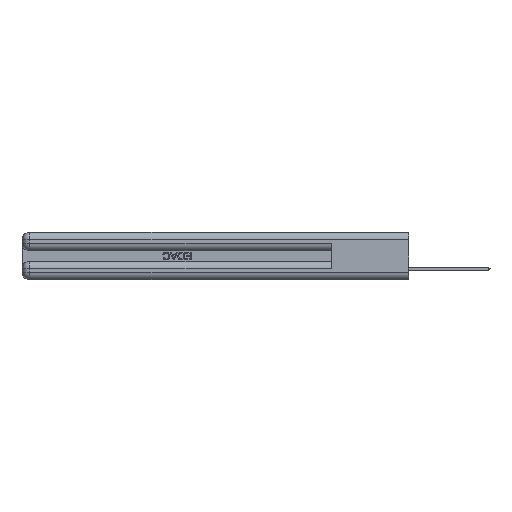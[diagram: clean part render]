
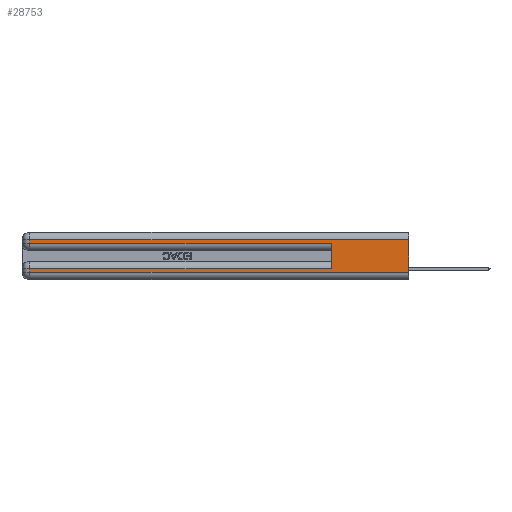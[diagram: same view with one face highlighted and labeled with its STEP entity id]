
A CAD part, left-side view. The second image highlights one B-rep face of the part: STEP entity #28753.
In plain terms, the highlighted planar face has unit normal (-1, 0, 0).
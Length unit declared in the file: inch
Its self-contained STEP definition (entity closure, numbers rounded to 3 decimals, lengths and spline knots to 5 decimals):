
#1187 = CARTESIAN_POINT ( 'NONE',  ( 0., 2.94, 0.31 ) ) ;
#1311 = VECTOR ( 'NONE', #47342, 39.37008 ) ;
#2061 = VERTEX_POINT ( 'NONE', #22111 ) ;
#3007 = CARTESIAN_POINT ( 'NONE',  ( 0., 0., 0.31 ) ) ;
#4517 = LINE ( 'NONE', #20306, #35977 ) ;
#5381 = ORIENTED_EDGE ( 'NONE', *, *, #28192, .T. ) ;
#7694 = DIRECTION ( 'NONE',  ( 0., 1., 0. ) ) ;
#9049 = EDGE_CURVE ( 'NONE', #15280, #13656, #18697, .T. ) ;
#9583 = EDGE_CURVE ( 'NONE', #20522, #40285, #17499, .T. ) ;
#11757 = PLANE ( 'NONE',  #12624 ) ;
#12578 = VECTOR ( 'NONE', #39625, 39.37008 ) ;
#12600 = EDGE_LOOP ( 'NONE', ( #22124, #5381, #37845, #44652, #40522, #27484, #21567, #27332 ) ) ;
#12624 = AXIS2_PLACEMENT_3D ( 'NONE', #39375, #23442, #51033 ) ;
#12992 = VERTEX_POINT ( 'NONE', #1187 ) ;
#13656 = VERTEX_POINT ( 'NONE', #49601 ) ;
#13977 = LINE ( 'NONE', #23666, #30680 ) ;
#15280 = VERTEX_POINT ( 'NONE', #34866 ) ;
#15989 = DIRECTION ( 'NONE',  ( 0., -1., 0. ) ) ;
#17499 = LINE ( 'NONE', #47185, #12578 ) ;
#18697 = LINE ( 'NONE', #21421, #29178 ) ;
#19286 = CARTESIAN_POINT ( 'NONE',  ( 0., 0., 0.06 ) ) ;
#20298 = CARTESIAN_POINT ( 'NONE',  ( 0., 0., 0.06 ) ) ;
#20306 = CARTESIAN_POINT ( 'NONE',  ( 0., 2.94, 0.37 ) ) ;
#20480 = DIRECTION ( 'NONE',  ( 0., 0., -1. ) ) ;
#20522 = VERTEX_POINT ( 'NONE', #38271 ) ;
#21421 = CARTESIAN_POINT ( 'NONE',  ( 0., 0., 0.085 ) ) ;
#21567 = ORIENTED_EDGE ( 'NONE', *, *, #30758, .T. ) ;
#22111 = CARTESIAN_POINT ( 'NONE',  ( 0., 2.94, 0.06 ) ) ;
#22124 = ORIENTED_EDGE ( 'NONE', *, *, #33357, .F. ) ;
#22220 = LINE ( 'NONE', #31991, #1311 ) ;
#22892 = EDGE_CURVE ( 'NONE', #15280, #40285, #22220, .T. ) ;
#23376 = VERTEX_POINT ( 'NONE', #3007 ) ;
#23442 = DIRECTION ( 'NONE',  ( 1., 0., 0. ) ) ;
#23666 = CARTESIAN_POINT ( 'NONE',  ( 0., 0., 0.31 ) ) ;
#24849 = DIRECTION ( 'NONE',  ( 0., 0., -1. ) ) ;
#25386 = DIRECTION ( 'NONE',  ( 0., 1., 0. ) ) ;
#25401 = CARTESIAN_POINT ( 'NONE',  ( 0., 2.94, 0.37 ) ) ;
#27332 = ORIENTED_EDGE ( 'NONE', *, *, #34290, .T. ) ;
#27484 = ORIENTED_EDGE ( 'NONE', *, *, #9049, .T. ) ;
#27805 = CARTESIAN_POINT ( 'NONE',  ( 0., 0.6, 0.285 ) ) ;
#28192 = EDGE_CURVE ( 'NONE', #23376, #12992, #13977, .T. ) ;
#28753 = ADVANCED_FACE ( 'NONE', ( #34325 ), #11757, .F. ) ;
#29178 = VECTOR ( 'NONE', #25386, 39.37008 ) ;
#29346 = CARTESIAN_POINT ( 'NONE',  ( 0., 0., 0.37 ) ) ;
#29542 = EDGE_CURVE ( 'NONE', #12992, #20522, #33020, .T. ) ;
#30680 = VECTOR ( 'NONE', #7694, 39.37008 ) ;
#30758 = EDGE_CURVE ( 'NONE', #13656, #2061, #4517, .T. ) ;
#31773 = VECTOR ( 'NONE', #45128, 39.37008 ) ;
#31991 = CARTESIAN_POINT ( 'NONE',  ( 0., 0.6, 0.145 ) ) ;
#33020 = LINE ( 'NONE', #25401, #31773 ) ;
#33357 = EDGE_CURVE ( 'NONE', #23376, #49647, #34187, .T. ) ;
#34187 = LINE ( 'NONE', #29346, #46556 ) ;
#34290 = EDGE_CURVE ( 'NONE', #2061, #49647, #49668, .T. ) ;
#34325 = FACE_OUTER_BOUND ( 'NONE', #12600, .T. ) ;
#34866 = CARTESIAN_POINT ( 'NONE',  ( 0., 0.6, 0.085 ) ) ;
#35977 = VECTOR ( 'NONE', #20480, 39.37008 ) ;
#37845 = ORIENTED_EDGE ( 'NONE', *, *, #29542, .T. ) ;
#38271 = CARTESIAN_POINT ( 'NONE',  ( 0., 2.94, 0.285 ) ) ;
#39375 = CARTESIAN_POINT ( 'NONE',  ( 0., 0., 0.37 ) ) ;
#39625 = DIRECTION ( 'NONE',  ( 0., -1., 0. ) ) ;
#39869 = VECTOR ( 'NONE', #15989, 39.37008 ) ;
#40285 = VERTEX_POINT ( 'NONE', #27805 ) ;
#40522 = ORIENTED_EDGE ( 'NONE', *, *, #22892, .F. ) ;
#44652 = ORIENTED_EDGE ( 'NONE', *, *, #9583, .T. ) ;
#45128 = DIRECTION ( 'NONE',  ( 0., 0., -1. ) ) ;
#46556 = VECTOR ( 'NONE', #24849, 39.37008 ) ;
#47185 = CARTESIAN_POINT ( 'NONE',  ( 0., 0., 0.285 ) ) ;
#47342 = DIRECTION ( 'NONE',  ( 0., 0., 1. ) ) ;
#49601 = CARTESIAN_POINT ( 'NONE',  ( 0., 2.94, 0.085 ) ) ;
#49647 = VERTEX_POINT ( 'NONE', #20298 ) ;
#49668 = LINE ( 'NONE', #19286, #39869 ) ;
#51033 = DIRECTION ( 'NONE',  ( 0., 0., -1. ) ) ;
